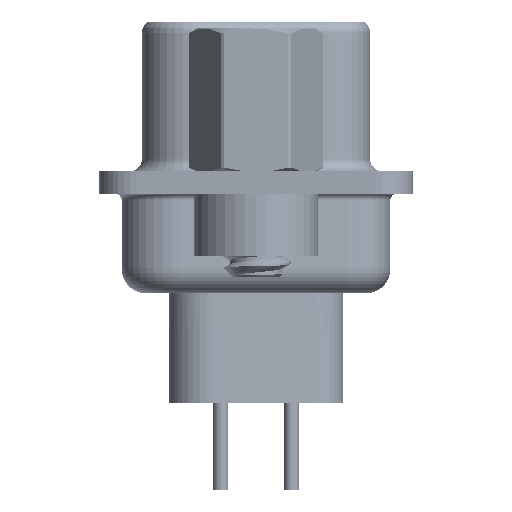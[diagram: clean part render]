
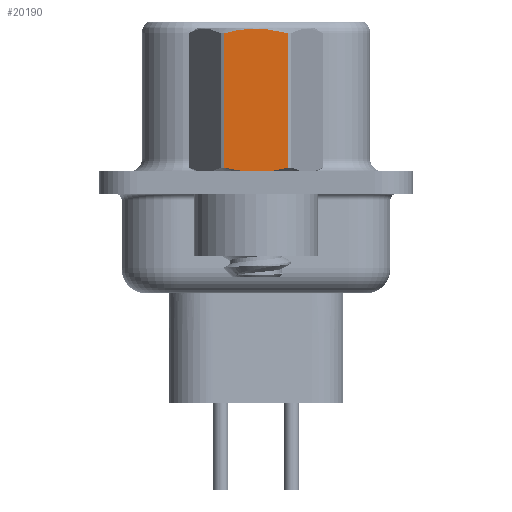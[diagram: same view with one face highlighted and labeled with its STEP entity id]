
A CAD part, left-side view. The second image highlights one B-rep face of the part: STEP entity #20190.
In plain terms, the highlighted planar face has unit normal (-1, 0, 0).
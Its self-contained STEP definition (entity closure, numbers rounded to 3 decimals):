
#10 = EDGE_LOOP ( 'NONE', ( #14384, #30496, #34496, #17014 ) ) ;
#306 = CARTESIAN_POINT ( 'NONE',  ( -2.381, 1.273, 0.602 ) ) ;
#1014 = CARTESIAN_POINT ( 'NONE',  ( -2.381, -0.858, 6.1 ) ) ;
#1390 = CARTESIAN_POINT ( 'NONE',  ( -2.381, -1.273, 5.998 ) ) ;
#2214 = CARTESIAN_POINT ( 'NONE',  ( -2.381, 1.273, 0.602 ) ) ;
#2251 = CARTESIAN_POINT ( 'NONE',  ( -2.381, 1.375, -3.8 ) ) ;
#4131 = CARTESIAN_POINT ( 'NONE',  ( -2.381, -1.273, 3.792 ) ) ;
#4201 = CARTESIAN_POINT ( 'NONE',  ( -2.381, -1.066, 6.054 ) ) ;
#4609 = CARTESIAN_POINT ( 'NONE',  ( -2.381, 1.273, 5.998 ) ) ;
#6779 = CARTESIAN_POINT ( 'NONE',  ( -2.381, 0.215, 0.418 ) ) ;
#7204 = CARTESIAN_POINT ( 'NONE',  ( -2.381, -0.432, 6.165 ) ) ;
#7440 = VECTOR ( 'NONE', #26937, 1000. ) ;
#7639 = LINE ( 'NONE', #4131, #7440 ) ;
#8389 = CARTESIAN_POINT ( 'NONE',  ( -2.381, -1.273, 5.998 ) ) ;
#8925 = VECTOR ( 'NONE', #26594, 1000. ) ;
#10186 = CARTESIAN_POINT ( 'NONE',  ( -2.381, 1.065, 6.054 ) ) ;
#11849 = VERTEX_POINT ( 'NONE', #306 ) ;
#12791 = CARTESIAN_POINT ( 'NONE',  ( -2.381, 0.428, 6.165 ) ) ;
#14083 = VERTEX_POINT ( 'NONE', #4609 ) ;
#14384 = ORIENTED_EDGE ( 'NONE', *, *, #25444, .T. ) ;
#15949 = EDGE_CURVE ( 'NONE', #19069, #22084, #7639, .T. ) ;
#16052 = CARTESIAN_POINT ( 'NONE',  ( -2.381, 1.065, 0.546 ) ) ;
#17014 = ORIENTED_EDGE ( 'NONE', *, *, #26142, .T. ) ;
#18703 = B_SPLINE_CURVE_WITH_KNOTS ( 'NONE', 3,
 ( #2214, #16052, #32179, #30260, #6779, #33435, #35172, #26774, #34980, #27471 ),
 .UNSPECIFIED., .F., .F.,
 ( 4, 2, 2, 2, 4 ),
 ( 0.003, 0.003, 0.004, 0.004, 0.005 ),
 .UNSPECIFIED. ) ;
#19069 = VERTEX_POINT ( 'NONE', #34373 ) ;
#20190 = ADVANCED_FACE ( 'NONE', ( #22251 ), #33465, .T. ) ;
#21283 = B_SPLINE_CURVE_WITH_KNOTS ( 'NONE', 3,
 ( #1390, #4201, #1014, #7204, #29978, #31715, #12791, #21395, #10186, #35219 ),
 .UNSPECIFIED., .F., .F.,
 ( 4, 2, 2, 2, 4 ),
 ( 0.001, 0.002, 0.002, 0.003, 0.004 ),
 .UNSPECIFIED. ) ;
#21395 = CARTESIAN_POINT ( 'NONE',  ( -2.381, 0.853, 6.101 ) ) ;
#22084 = VERTEX_POINT ( 'NONE', #8389 ) ;
#22251 = FACE_OUTER_BOUND ( 'NONE', #10, .T. ) ;
#25247 = DIRECTION ( 'NONE',  ( -1., 0., 0. ) ) ;
#25444 = EDGE_CURVE ( 'NONE', #11849, #19069, #18703, .T. ) ;
#26142 = EDGE_CURVE ( 'NONE', #14083, #11849, #35359, .T. ) ;
#26594 = DIRECTION ( 'NONE',  ( 0., 0., -1. ) ) ;
#26774 = CARTESIAN_POINT ( 'NONE',  ( -2.381, -0.858, 0.5 ) ) ;
#26937 = DIRECTION ( 'NONE',  ( 0., 0., 1. ) ) ;
#27434 = EDGE_CURVE ( 'NONE', #22084, #14083, #21283, .T. ) ;
#27471 = CARTESIAN_POINT ( 'NONE',  ( -2.381, -1.273, 0.602 ) ) ;
#29978 = CARTESIAN_POINT ( 'NONE',  ( -2.381, -0.215, 6.182 ) ) ;
#30260 = CARTESIAN_POINT ( 'NONE',  ( -2.381, 0.428, 0.435 ) ) ;
#30496 = ORIENTED_EDGE ( 'NONE', *, *, #15949, .T. ) ;
#31715 = CARTESIAN_POINT ( 'NONE',  ( -2.381, 0.215, 6.182 ) ) ;
#32179 = CARTESIAN_POINT ( 'NONE',  ( -2.381, 0.853, 0.499 ) ) ;
#32370 = CARTESIAN_POINT ( 'NONE',  ( -2.381, 1.273, 3.792 ) ) ;
#33435 = CARTESIAN_POINT ( 'NONE',  ( -2.381, -0.215, 0.418 ) ) ;
#33465 = PLANE ( 'NONE',  #36306 ) ;
#33834 = DIRECTION ( 'NONE',  ( 0., -1., 0. ) ) ;
#34373 = CARTESIAN_POINT ( 'NONE',  ( -2.381, -1.273, 0.602 ) ) ;
#34496 = ORIENTED_EDGE ( 'NONE', *, *, #27434, .T. ) ;
#34980 = CARTESIAN_POINT ( 'NONE',  ( -2.381, -1.066, 0.546 ) ) ;
#35172 = CARTESIAN_POINT ( 'NONE',  ( -2.381, -0.432, 0.435 ) ) ;
#35219 = CARTESIAN_POINT ( 'NONE',  ( -2.381, 1.273, 5.998 ) ) ;
#35359 = LINE ( 'NONE', #32370, #8925 ) ;
#36306 = AXIS2_PLACEMENT_3D ( 'NONE', #2251, #25247, #33834 ) ;
